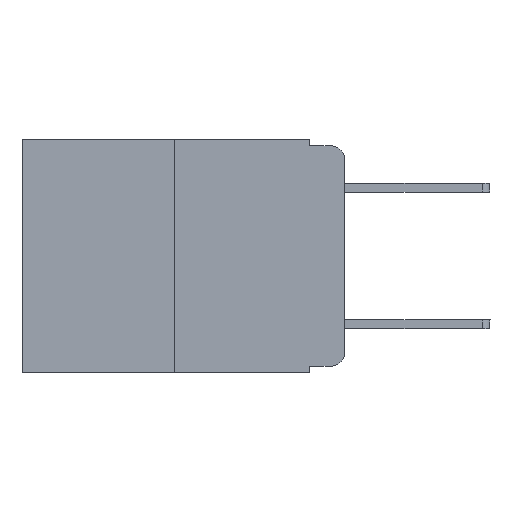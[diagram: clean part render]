
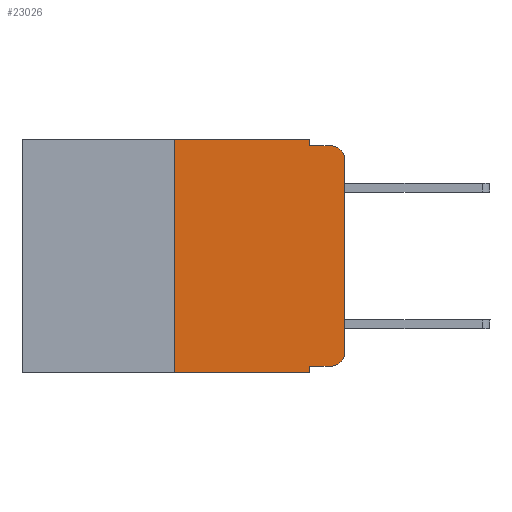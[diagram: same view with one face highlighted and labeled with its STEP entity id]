
A CAD part, left-side view. The second image highlights one B-rep face of the part: STEP entity #23026.
In plain terms, the highlighted planar face has unit normal (-1, 0, 0).
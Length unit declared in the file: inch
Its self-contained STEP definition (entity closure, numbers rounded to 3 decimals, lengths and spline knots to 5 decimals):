
#6 = CARTESIAN_POINT ( 'NONE',  ( 0., 0.02, -0.01 ) ) ;
#335 = DIRECTION ( 'NONE',  ( 0., 0., -1. ) ) ;
#490 = DIRECTION ( 'NONE',  ( 0., -1., 0. ) ) ;
#651 = EDGE_CURVE ( 'NONE', #4155, #14214, #19968, .T. ) ;
#688 = VECTOR ( 'NONE', #14224, 39.37008 ) ;
#730 = CARTESIAN_POINT ( 'NONE',  ( 0., 0.473, -0.343 ) ) ;
#1061 = EDGE_CURVE ( 'NONE', #23370, #11914, #14155, .T. ) ;
#1110 = VERTEX_POINT ( 'NONE', #23889 ) ;
#1265 = VECTOR ( 'NONE', #490, 39.37008 ) ;
#1728 = DIRECTION ( 'NONE',  ( 0., -1., 0. ) ) ;
#1868 = CARTESIAN_POINT ( 'NONE',  ( 0., 0.051, -0.333 ) ) ;
#1888 = CARTESIAN_POINT ( 'NONE',  ( 0., 0.473, 0. ) ) ;
#3182 = VERTEX_POINT ( 'NONE', #4415 ) ;
#3442 = LINE ( 'NONE', #4124, #18772 ) ;
#3867 = LINE ( 'NONE', #19645, #688 ) ;
#4124 = CARTESIAN_POINT ( 'NONE',  ( 0., 0.051, -0.01 ) ) ;
#4155 = VERTEX_POINT ( 'NONE', #23665 ) ;
#4415 = CARTESIAN_POINT ( 'NONE',  ( 0., 0.25, -0.343 ) ) ;
#4438 = LINE ( 'NONE', #730, #1265 ) ;
#4514 = CIRCLE ( 'NONE', #9850, 0.02 ) ;
#5184 = DIRECTION ( 'NONE',  ( -1., 0., 0. ) ) ;
#5452 = DIRECTION ( 'NONE',  ( 0., -1., 0. ) ) ;
#5650 = LINE ( 'NONE', #20684, #6790 ) ;
#5797 = EDGE_CURVE ( 'NONE', #23302, #1110, #16942, .T. ) ;
#5810 = CARTESIAN_POINT ( 'NONE',  ( 0., 0.02, -0.333 ) ) ;
#6109 = VECTOR ( 'NONE', #9783, 39.37008 ) ;
#6310 = FACE_OUTER_BOUND ( 'NONE', #9744, .T. ) ;
#6778 = EDGE_CURVE ( 'NONE', #1110, #21059, #3867, .T. ) ;
#6790 = VECTOR ( 'NONE', #15177, 39.37008 ) ;
#6949 = ORIENTED_EDGE ( 'NONE', *, *, #15953, .T. ) ;
#7450 = PLANE ( 'NONE',  #19387 ) ;
#7533 = DIRECTION ( 'NONE',  ( 1., 0., 0. ) ) ;
#7697 = CARTESIAN_POINT ( 'NONE',  ( 0., 0.473, 0. ) ) ;
#7759 = VERTEX_POINT ( 'NONE', #8238 ) ;
#8238 = CARTESIAN_POINT ( 'NONE',  ( 0., 0., -0.313 ) ) ;
#8889 = EDGE_CURVE ( 'NONE', #3182, #23302, #19134, .T. ) ;
#9744 = EDGE_LOOP ( 'NONE', ( #14206, #21690, #13997, #13897, #23009, #18302, #20602, #20303, #14285, #6949 ) ) ;
#9782 = DIRECTION ( 'NONE',  ( 0., -1., 0. ) ) ;
#9783 = DIRECTION ( 'NONE',  ( 0., 0., 1. ) ) ;
#9850 = AXIS2_PLACEMENT_3D ( 'NONE', #20049, #5184, #12452 ) ;
#10347 = CARTESIAN_POINT ( 'NONE',  ( 0., 0.051, -0.01 ) ) ;
#10389 = DIRECTION ( 'NONE',  ( 0., 0., -1. ) ) ;
#10639 = EDGE_CURVE ( 'NONE', #23370, #23654, #16388, .T. ) ;
#11358 = DIRECTION ( 'NONE',  ( 0., 0., -1. ) ) ;
#11436 = DIRECTION ( 'NONE',  ( -1., 0., 0. ) ) ;
#11914 = VERTEX_POINT ( 'NONE', #5810 ) ;
#12204 = CARTESIAN_POINT ( 'NONE',  ( 0., 0.25, 0. ) ) ;
#12452 = DIRECTION ( 'NONE',  ( 0., 0., -1. ) ) ;
#13171 = VECTOR ( 'NONE', #1728, 39.37008 ) ;
#13897 = ORIENTED_EDGE ( 'NONE', *, *, #6778, .F. ) ;
#13997 = ORIENTED_EDGE ( 'NONE', *, *, #20892, .F. ) ;
#14155 = LINE ( 'NONE', #1868, #21992 ) ;
#14206 = ORIENTED_EDGE ( 'NONE', *, *, #16897, .T. ) ;
#14214 = VERTEX_POINT ( 'NONE', #6 ) ;
#14224 = DIRECTION ( 'NONE',  ( 0., 0., -1. ) ) ;
#14285 = ORIENTED_EDGE ( 'NONE', *, *, #1061, .T. ) ;
#14658 = CARTESIAN_POINT ( 'NONE',  ( 0., 0.02, -0.03 ) ) ;
#15177 = DIRECTION ( 'NONE',  ( 0., 0., 1. ) ) ;
#15245 = CARTESIAN_POINT ( 'NONE',  ( 0., 0.051, -0.343 ) ) ;
#15783 = CARTESIAN_POINT ( 'NONE',  ( 0., 0.051, 0. ) ) ;
#15953 = EDGE_CURVE ( 'NONE', #11914, #7759, #4514, .T. ) ;
#16388 = LINE ( 'NONE', #15783, #22785 ) ;
#16897 = EDGE_CURVE ( 'NONE', #7759, #4155, #5650, .T. ) ;
#16942 = LINE ( 'NONE', #1888, #13171 ) ;
#18223 = EDGE_CURVE ( 'NONE', #3182, #23654, #4438, .T. ) ;
#18302 = ORIENTED_EDGE ( 'NONE', *, *, #8889, .F. ) ;
#18723 = AXIS2_PLACEMENT_3D ( 'NONE', #14658, #11436, #11358 ) ;
#18772 = VECTOR ( 'NONE', #9782, 39.37008 ) ;
#19134 = LINE ( 'NONE', #20844, #6109 ) ;
#19387 = AXIS2_PLACEMENT_3D ( 'NONE', #7697, #7533, #335 ) ;
#19645 = CARTESIAN_POINT ( 'NONE',  ( 0., 0.051, 0. ) ) ;
#19968 = CIRCLE ( 'NONE', #18723, 0.02 ) ;
#20049 = CARTESIAN_POINT ( 'NONE',  ( 0., 0.02, -0.313 ) ) ;
#20303 = ORIENTED_EDGE ( 'NONE', *, *, #10639, .F. ) ;
#20602 = ORIENTED_EDGE ( 'NONE', *, *, #18223, .T. ) ;
#20684 = CARTESIAN_POINT ( 'NONE',  ( 0., 0., 0. ) ) ;
#20844 = CARTESIAN_POINT ( 'NONE',  ( 0., 0.25, 0. ) ) ;
#20892 = EDGE_CURVE ( 'NONE', #21059, #14214, #3442, .T. ) ;
#21059 = VERTEX_POINT ( 'NONE', #10347 ) ;
#21690 = ORIENTED_EDGE ( 'NONE', *, *, #651, .T. ) ;
#21992 = VECTOR ( 'NONE', #5452, 39.37008 ) ;
#22785 = VECTOR ( 'NONE', #10389, 39.37008 ) ;
#23009 = ORIENTED_EDGE ( 'NONE', *, *, #5797, .F. ) ;
#23026 = ADVANCED_FACE ( 'NONE', ( #6310 ), #7450, .F. ) ;
#23302 = VERTEX_POINT ( 'NONE', #12204 ) ;
#23370 = VERTEX_POINT ( 'NONE', #23754 ) ;
#23654 = VERTEX_POINT ( 'NONE', #15245 ) ;
#23665 = CARTESIAN_POINT ( 'NONE',  ( 0., 0., -0.03 ) ) ;
#23754 = CARTESIAN_POINT ( 'NONE',  ( 0., 0.051, -0.333 ) ) ;
#23889 = CARTESIAN_POINT ( 'NONE',  ( 0., 0.051, 0. ) ) ;
